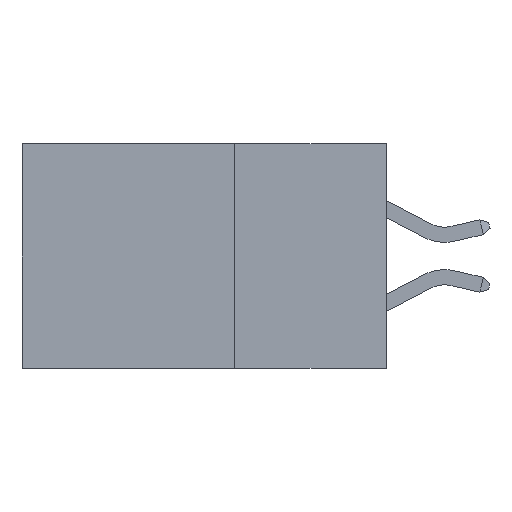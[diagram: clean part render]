
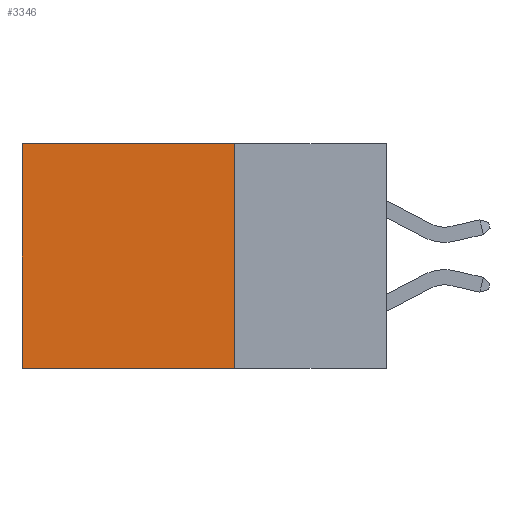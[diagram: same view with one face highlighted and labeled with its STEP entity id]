
A CAD part, left-side view. The second image highlights one B-rep face of the part: STEP entity #3346.
In plain terms, the highlighted planar face has unit normal (-1, 0, 0).
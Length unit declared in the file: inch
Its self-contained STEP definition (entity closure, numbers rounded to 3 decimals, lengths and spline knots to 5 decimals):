
#317 = VECTOR ( 'NONE', #7282, 39.37008 ) ;
#386 = VERTEX_POINT ( 'NONE', #5821 ) ;
#824 = DIRECTION ( 'NONE',  ( 1., 0., 0. ) ) ;
#909 = EDGE_LOOP ( 'NONE', ( #3335, #3654, #11183, #1875 ) ) ;
#1779 = CARTESIAN_POINT ( 'NONE',  ( 0.2615, 0.25, 0. ) ) ;
#1875 = ORIENTED_EDGE ( 'NONE', *, *, #7521, .T. ) ;
#2955 = DIRECTION ( 'NONE',  ( 0., 0., -1. ) ) ;
#3283 = VERTEX_POINT ( 'NONE', #5844 ) ;
#3335 = ORIENTED_EDGE ( 'NONE', *, *, #4741, .T. ) ;
#3346 = ADVANCED_FACE ( 'NONE', ( #5260 ), #9000, .F. ) ;
#3392 = CARTESIAN_POINT ( 'NONE',  ( 0.2615, 0.6, 0. ) ) ;
#3654 = ORIENTED_EDGE ( 'NONE', *, *, #6214, .F. ) ;
#4664 = CARTESIAN_POINT ( 'NONE',  ( 0.2615, 0.25, -0.37 ) ) ;
#4741 = EDGE_CURVE ( 'NONE', #4895, #386, #11099, .T. ) ;
#4895 = VERTEX_POINT ( 'NONE', #3392 ) ;
#5243 = VECTOR ( 'NONE', #8055, 39.37008 ) ;
#5260 = FACE_OUTER_BOUND ( 'NONE', #909, .T. ) ;
#5530 = DIRECTION ( 'NONE',  ( 0., 0., -1. ) ) ;
#5821 = CARTESIAN_POINT ( 'NONE',  ( 0.2615, 0.6, -0.37 ) ) ;
#5844 = CARTESIAN_POINT ( 'NONE',  ( 0.2615, 0.25, -0.37 ) ) ;
#6214 = EDGE_CURVE ( 'NONE', #3283, #386, #10010, .T. ) ;
#6381 = LINE ( 'NONE', #1779, #5243 ) ;
#6648 = VERTEX_POINT ( 'NONE', #7270 ) ;
#6670 = AXIS2_PLACEMENT_3D ( 'NONE', #7068, #824, #5530 ) ;
#7022 = VECTOR ( 'NONE', #2955, 39.37008 ) ;
#7068 = CARTESIAN_POINT ( 'NONE',  ( 0.2615, 0.25, -0.37 ) ) ;
#7270 = CARTESIAN_POINT ( 'NONE',  ( 0.2615, 0.25, 0. ) ) ;
#7282 = DIRECTION ( 'NONE',  ( 0., 1., 0. ) ) ;
#7521 = EDGE_CURVE ( 'NONE', #6648, #4895, #6381, .T. ) ;
#8055 = DIRECTION ( 'NONE',  ( 0., 1., 0. ) ) ;
#8131 = CARTESIAN_POINT ( 'NONE',  ( 0.2615, 0.25, -0.37 ) ) ;
#8265 = CARTESIAN_POINT ( 'NONE',  ( 0.2615, 0.6, -0.37 ) ) ;
#8782 = VECTOR ( 'NONE', #9290, 39.37008 ) ;
#8928 = LINE ( 'NONE', #8131, #7022 ) ;
#9000 = PLANE ( 'NONE',  #6670 ) ;
#9290 = DIRECTION ( 'NONE',  ( 0., 0., -1. ) ) ;
#10010 = LINE ( 'NONE', #4664, #317 ) ;
#10896 = EDGE_CURVE ( 'NONE', #6648, #3283, #8928, .T. ) ;
#11099 = LINE ( 'NONE', #8265, #8782 ) ;
#11183 = ORIENTED_EDGE ( 'NONE', *, *, #10896, .F. ) ;
